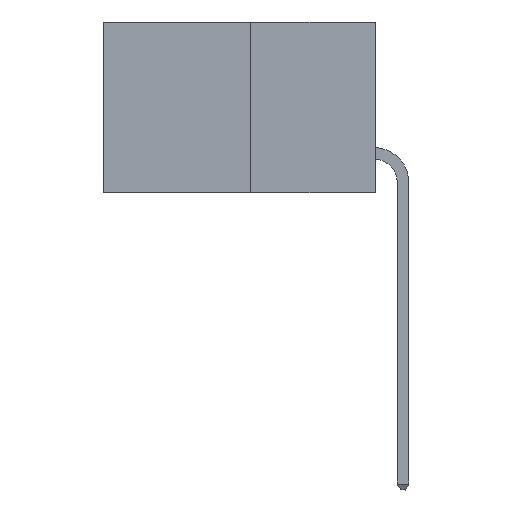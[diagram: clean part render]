
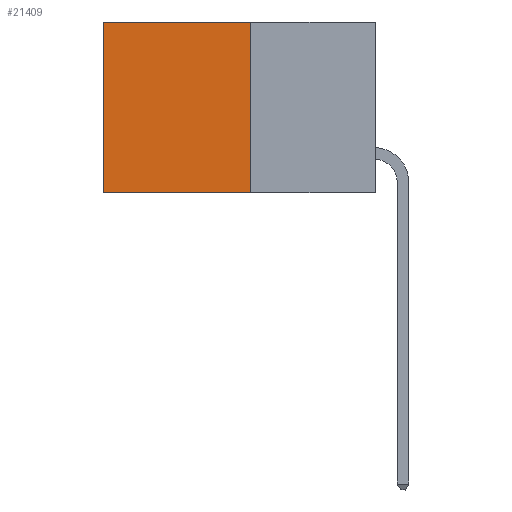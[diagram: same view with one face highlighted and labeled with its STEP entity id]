
A CAD part, left-side view. The second image highlights one B-rep face of the part: STEP entity #21409.
In plain terms, the highlighted planar face has unit normal (-1, 0, 0).
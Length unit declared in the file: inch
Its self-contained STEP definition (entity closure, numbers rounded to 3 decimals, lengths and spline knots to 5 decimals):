
#269 = EDGE_LOOP ( 'NONE', ( #4447, #21982, #19097, #26293 ) ) ;
#1364 = LINE ( 'NONE', #28735, #18935 ) ;
#1499 = VERTEX_POINT ( 'NONE', #20767 ) ;
#2613 = VERTEX_POINT ( 'NONE', #27522 ) ;
#4147 = LINE ( 'NONE', #23962, #15657 ) ;
#4447 = ORIENTED_EDGE ( 'NONE', *, *, #17952, .T. ) ;
#5026 = VECTOR ( 'NONE', #11766, 39.37008 ) ;
#5993 = DIRECTION ( 'NONE',  ( 0., 0., -1. ) ) ;
#6951 = FACE_OUTER_BOUND ( 'NONE', #269, .T. ) ;
#8264 = LINE ( 'NONE', #21918, #19694 ) ;
#8308 = CARTESIAN_POINT ( 'NONE',  ( 0.277, 0.27, -0.37 ) ) ;
#9462 = CARTESIAN_POINT ( 'NONE',  ( 0.277, 0.27, -0.37 ) ) ;
#10953 = EDGE_CURVE ( 'NONE', #2613, #21374, #8264, .T. ) ;
#11560 = DIRECTION ( 'NONE',  ( 1., 0., 0. ) ) ;
#11766 = DIRECTION ( 'NONE',  ( 0., 0., -1. ) ) ;
#12274 = CARTESIAN_POINT ( 'NONE',  ( 0.277, 0.27, -0.37 ) ) ;
#15123 = DIRECTION ( 'NONE',  ( 0., 1., 0. ) ) ;
#15627 = AXIS2_PLACEMENT_3D ( 'NONE', #12274, #11560, #27510 ) ;
#15657 = VECTOR ( 'NONE', #26228, 39.37008 ) ;
#16992 = EDGE_CURVE ( 'NONE', #2613, #28745, #23284, .T. ) ;
#17952 = EDGE_CURVE ( 'NONE', #21374, #1499, #1364, .T. ) ;
#18935 = VECTOR ( 'NONE', #5993, 39.37008 ) ;
#19097 = ORIENTED_EDGE ( 'NONE', *, *, #16992, .F. ) ;
#19143 = EDGE_CURVE ( 'NONE', #28745, #1499, #4147, .T. ) ;
#19694 = VECTOR ( 'NONE', #15123, 39.37008 ) ;
#20767 = CARTESIAN_POINT ( 'NONE',  ( 0.277, 0.59, -0.37 ) ) ;
#21374 = VERTEX_POINT ( 'NONE', #25030 ) ;
#21409 = ADVANCED_FACE ( 'NONE', ( #6951 ), #25222, .F. ) ;
#21918 = CARTESIAN_POINT ( 'NONE',  ( 0.277, 0.27, 0. ) ) ;
#21982 = ORIENTED_EDGE ( 'NONE', *, *, #19143, .F. ) ;
#23284 = LINE ( 'NONE', #9462, #5026 ) ;
#23962 = CARTESIAN_POINT ( 'NONE',  ( 0.277, 0.27, -0.37 ) ) ;
#25030 = CARTESIAN_POINT ( 'NONE',  ( 0.277, 0.59, 0. ) ) ;
#25222 = PLANE ( 'NONE',  #15627 ) ;
#26228 = DIRECTION ( 'NONE',  ( 0., 1., 0. ) ) ;
#26293 = ORIENTED_EDGE ( 'NONE', *, *, #10953, .T. ) ;
#27510 = DIRECTION ( 'NONE',  ( 0., 0., -1. ) ) ;
#27522 = CARTESIAN_POINT ( 'NONE',  ( 0.277, 0.27, 0. ) ) ;
#28735 = CARTESIAN_POINT ( 'NONE',  ( 0.277, 0.59, -0.37 ) ) ;
#28745 = VERTEX_POINT ( 'NONE', #8308 ) ;
